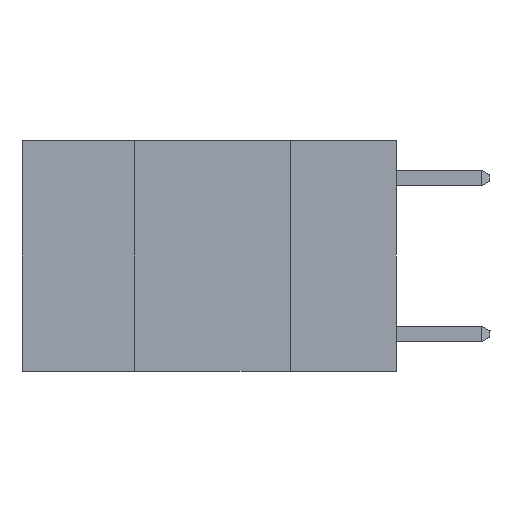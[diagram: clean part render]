
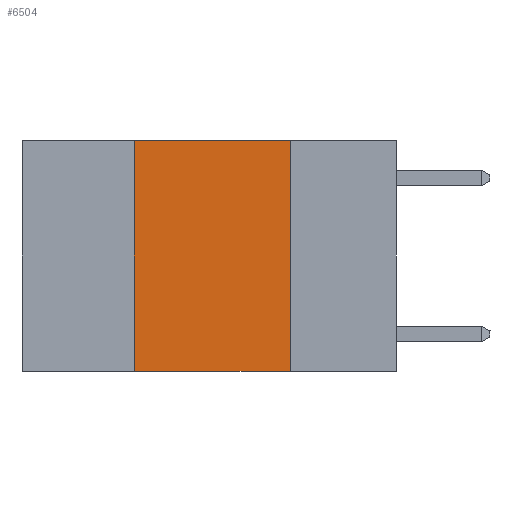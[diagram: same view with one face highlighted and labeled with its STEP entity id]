
A CAD part, left-side view. The second image highlights one B-rep face of the part: STEP entity #6504.
In plain terms, the highlighted planar face has unit normal (-1, 0, 0).
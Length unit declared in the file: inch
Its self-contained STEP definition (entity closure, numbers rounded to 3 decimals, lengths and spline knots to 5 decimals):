
#150 = EDGE_CURVE ( 'NONE', #437, #1724, #1036, .T. ) ;
#409 = VERTEX_POINT ( 'NONE', #6318 ) ;
#437 = VERTEX_POINT ( 'NONE', #4835 ) ;
#476 = CARTESIAN_POINT ( 'NONE',  ( 0., 0.17, -0.37 ) ) ;
#947 = DIRECTION ( 'NONE',  ( 0., -1., 0. ) ) ;
#1036 = LINE ( 'NONE', #9446, #9514 ) ;
#1100 = CARTESIAN_POINT ( 'NONE',  ( 0., 0.6, 0. ) ) ;
#1602 = CARTESIAN_POINT ( 'NONE',  ( 0., 0.42, -0.37 ) ) ;
#1607 = EDGE_CURVE ( 'NONE', #3506, #409, #2086, .T. ) ;
#1721 = DIRECTION ( 'NONE',  ( 0., 0., -1. ) ) ;
#1724 = VERTEX_POINT ( 'NONE', #476 ) ;
#1993 = DIRECTION ( 'NONE',  ( 0., 0., 1. ) ) ;
#2086 = LINE ( 'NONE', #2119, #8346 ) ;
#2119 = CARTESIAN_POINT ( 'NONE',  ( 0., 0.42, 0. ) ) ;
#2875 = FACE_OUTER_BOUND ( 'NONE', #6810, .T. ) ;
#3142 = ORIENTED_EDGE ( 'NONE', *, *, #3844, .F. ) ;
#3150 = ORIENTED_EDGE ( 'NONE', *, *, #5346, .T. ) ;
#3506 = VERTEX_POINT ( 'NONE', #1602 ) ;
#3588 = LINE ( 'NONE', #4388, #5345 ) ;
#3681 = ORIENTED_EDGE ( 'NONE', *, *, #1607, .F. ) ;
#3844 = EDGE_CURVE ( 'NONE', #409, #437, #8140, .T. ) ;
#4286 = CARTESIAN_POINT ( 'NONE',  ( 0., 0.6, 0. ) ) ;
#4388 = CARTESIAN_POINT ( 'NONE',  ( 0., 0.6, -0.37 ) ) ;
#4835 = CARTESIAN_POINT ( 'NONE',  ( 0., 0.17, 0. ) ) ;
#5345 = VECTOR ( 'NONE', #947, 39.37008 ) ;
#5346 = EDGE_CURVE ( 'NONE', #3506, #1724, #3588, .T. ) ;
#6318 = CARTESIAN_POINT ( 'NONE',  ( 0., 0.42, 0. ) ) ;
#6504 = ADVANCED_FACE ( 'NONE', ( #2875 ), #10091, .F. ) ;
#6810 = EDGE_LOOP ( 'NONE', ( #9445, #3142, #3681, #3150 ) ) ;
#6866 = DIRECTION ( 'NONE',  ( 1., 0., 0. ) ) ;
#7082 = DIRECTION ( 'NONE',  ( 0., -1., 0. ) ) ;
#8140 = LINE ( 'NONE', #1100, #10279 ) ;
#8170 = AXIS2_PLACEMENT_3D ( 'NONE', #4286, #6866, #1721 ) ;
#8346 = VECTOR ( 'NONE', #1993, 39.37008 ) ;
#9445 = ORIENTED_EDGE ( 'NONE', *, *, #150, .F. ) ;
#9446 = CARTESIAN_POINT ( 'NONE',  ( 0., 0.17, 0. ) ) ;
#9514 = VECTOR ( 'NONE', #10657, 39.37008 ) ;
#10091 = PLANE ( 'NONE',  #8170 ) ;
#10279 = VECTOR ( 'NONE', #7082, 39.37008 ) ;
#10657 = DIRECTION ( 'NONE',  ( 0., 0., -1. ) ) ;
